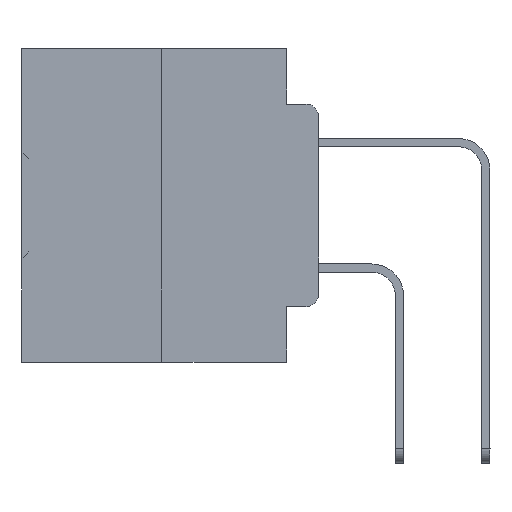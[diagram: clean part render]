
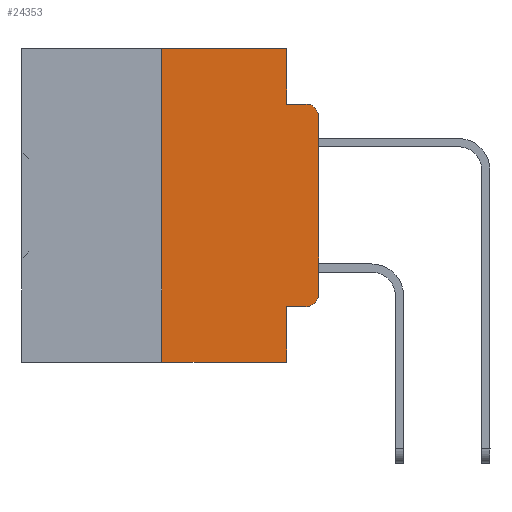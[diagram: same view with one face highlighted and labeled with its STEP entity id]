
A CAD part, left-side view. The second image highlights one B-rep face of the part: STEP entity #24353.
In plain terms, the highlighted planar face has unit normal (-1, 0, 0).
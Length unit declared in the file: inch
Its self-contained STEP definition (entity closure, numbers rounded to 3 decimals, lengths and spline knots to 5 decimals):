
#360 = ORIENTED_EDGE ( 'NONE', *, *, #14744, .F. ) ;
#1172 = ORIENTED_EDGE ( 'NONE', *, *, #17525, .T. ) ;
#1240 = ORIENTED_EDGE ( 'NONE', *, *, #19256, .T. ) ;
#1811 = DIRECTION ( 'NONE',  ( 0., -1., 0. ) ) ;
#2432 = DIRECTION ( 'NONE',  ( 0., 0., -1. ) ) ;
#2628 = ORIENTED_EDGE ( 'NONE', *, *, #6548, .T. ) ;
#3210 = ORIENTED_EDGE ( 'NONE', *, *, #6159, .T. ) ;
#3974 = CARTESIAN_POINT ( 'NONE',  ( 0., 0.051, 0. ) ) ;
#5320 = VERTEX_POINT ( 'NONE', #37767 ) ;
#5536 = VECTOR ( 'NONE', #11918, 39.37008 ) ;
#5666 = AXIS2_PLACEMENT_3D ( 'NONE', #34606, #37260, #12743 ) ;
#6159 = EDGE_CURVE ( 'NONE', #8242, #31587, #16073, .T. ) ;
#6332 = CARTESIAN_POINT ( 'NONE',  ( 0., 0.051, 0. ) ) ;
#6548 = EDGE_CURVE ( 'NONE', #24073, #8242, #27234, .T. ) ;
#6942 = CARTESIAN_POINT ( 'NONE',  ( 0., 0.051, -0.4115 ) ) ;
#7575 = CARTESIAN_POINT ( 'NONE',  ( 0., 0.25, 0. ) ) ;
#8065 = LINE ( 'NONE', #23955, #5536 ) ;
#8242 = VERTEX_POINT ( 'NONE', #32016 ) ;
#8620 = VECTOR ( 'NONE', #15705, 39.37008 ) ;
#9000 = VERTEX_POINT ( 'NONE', #39916 ) ;
#9559 = ORIENTED_EDGE ( 'NONE', *, *, #33309, .F. ) ;
#9646 = VECTOR ( 'NONE', #20033, 39.37008 ) ;
#9676 = CIRCLE ( 'NONE', #37721, 0.02 ) ;
#9790 = DIRECTION ( 'NONE',  ( 0., 0., -1. ) ) ;
#10258 = CARTESIAN_POINT ( 'NONE',  ( 0., 0.051, 0. ) ) ;
#10479 = LINE ( 'NONE', #3974, #38012 ) ;
#11151 = CARTESIAN_POINT ( 'NONE',  ( 0., 0.02, -0.0885 ) ) ;
#11415 = ORIENTED_EDGE ( 'NONE', *, *, #15819, .F. ) ;
#11901 = VERTEX_POINT ( 'NONE', #13279 ) ;
#11918 = DIRECTION ( 'NONE',  ( 0., 0., 1. ) ) ;
#12448 = CARTESIAN_POINT ( 'NONE',  ( 0., 0.02, -0.1085 ) ) ;
#12743 = DIRECTION ( 'NONE',  ( 0., 0., -1. ) ) ;
#13279 = CARTESIAN_POINT ( 'NONE',  ( 0., 0.051, -0.5 ) ) ;
#14744 = EDGE_CURVE ( 'NONE', #30869, #9000, #16304, .T. ) ;
#15273 = CARTESIAN_POINT ( 'NONE',  ( 0., 0., -0.3915 ) ) ;
#15677 = DIRECTION ( 'NONE',  ( 0., -1., 0. ) ) ;
#15705 = DIRECTION ( 'NONE',  ( 0., 0., -1. ) ) ;
#15819 = EDGE_CURVE ( 'NONE', #24073, #11901, #10479, .T. ) ;
#16073 = CIRCLE ( 'NONE', #5666, 0.02 ) ;
#16304 = LINE ( 'NONE', #6332, #8620 ) ;
#17028 = VERTEX_POINT ( 'NONE', #40156 ) ;
#17193 = LINE ( 'NONE', #29066, #34954 ) ;
#17505 = LINE ( 'NONE', #23035, #19625 ) ;
#17525 = EDGE_CURVE ( 'NONE', #31587, #17028, #8065, .T. ) ;
#18326 = VECTOR ( 'NONE', #15677, 39.37008 ) ;
#19256 = EDGE_CURVE ( 'NONE', #27452, #11901, #17193, .T. ) ;
#19332 = VECTOR ( 'NONE', #23729, 39.37008 ) ;
#19625 = VECTOR ( 'NONE', #1811, 39.37008 ) ;
#20033 = DIRECTION ( 'NONE',  ( 0., 0., 1. ) ) ;
#20353 = EDGE_LOOP ( 'NONE', ( #1172, #33511, #40323, #360, #9559, #34715, #1240, #11415, #2628, #3210 ) ) ;
#21201 = DIRECTION ( 'NONE',  ( 1., 0., 0. ) ) ;
#22099 = VERTEX_POINT ( 'NONE', #11151 ) ;
#23035 = CARTESIAN_POINT ( 'NONE',  ( 0., 0.473, 0. ) ) ;
#23729 = DIRECTION ( 'NONE',  ( 0., -1., 0. ) ) ;
#23955 = CARTESIAN_POINT ( 'NONE',  ( 0., 0., 0. ) ) ;
#24073 = VERTEX_POINT ( 'NONE', #6942 ) ;
#24353 = ADVANCED_FACE ( 'NONE', ( #38392 ), #35305, .F. ) ;
#24676 = CARTESIAN_POINT ( 'NONE',  ( 0., 0.051, -0.0885 ) ) ;
#27234 = LINE ( 'NONE', #36403, #19332 ) ;
#27452 = VERTEX_POINT ( 'NONE', #33228 ) ;
#28889 = DIRECTION ( 'NONE',  ( 0., 0., -1. ) ) ;
#29066 = CARTESIAN_POINT ( 'NONE',  ( 0., 0.473, -0.5 ) ) ;
#29199 = CARTESIAN_POINT ( 'NONE',  ( 0., 0.473, 0. ) ) ;
#29661 = DIRECTION ( 'NONE',  ( 0., -1., 0. ) ) ;
#30869 = VERTEX_POINT ( 'NONE', #10258 ) ;
#31556 = EDGE_CURVE ( 'NONE', #9000, #22099, #33677, .T. ) ;
#31587 = VERTEX_POINT ( 'NONE', #15273 ) ;
#32016 = CARTESIAN_POINT ( 'NONE',  ( 0., 0.02, -0.4115 ) ) ;
#33228 = CARTESIAN_POINT ( 'NONE',  ( 0., 0.25, -0.5 ) ) ;
#33309 = EDGE_CURVE ( 'NONE', #5320, #30869, #17505, .T. ) ;
#33511 = ORIENTED_EDGE ( 'NONE', *, *, #37702, .T. ) ;
#33677 = LINE ( 'NONE', #24676, #18326 ) ;
#34606 = CARTESIAN_POINT ( 'NONE',  ( 0., 0.02, -0.3915 ) ) ;
#34715 = ORIENTED_EDGE ( 'NONE', *, *, #37468, .F. ) ;
#34930 = AXIS2_PLACEMENT_3D ( 'NONE', #29199, #21201, #2432 ) ;
#34954 = VECTOR ( 'NONE', #29661, 39.37008 ) ;
#35305 = PLANE ( 'NONE',  #34930 ) ;
#35545 = LINE ( 'NONE', #7575, #9646 ) ;
#36403 = CARTESIAN_POINT ( 'NONE',  ( 0., 0.051, -0.4115 ) ) ;
#37260 = DIRECTION ( 'NONE',  ( -1., 0., 0. ) ) ;
#37468 = EDGE_CURVE ( 'NONE', #27452, #5320, #35545, .T. ) ;
#37570 = DIRECTION ( 'NONE',  ( -1., 0., 0. ) ) ;
#37702 = EDGE_CURVE ( 'NONE', #17028, #22099, #9676, .T. ) ;
#37721 = AXIS2_PLACEMENT_3D ( 'NONE', #12448, #37570, #9790 ) ;
#37767 = CARTESIAN_POINT ( 'NONE',  ( 0., 0.25, 0. ) ) ;
#38012 = VECTOR ( 'NONE', #28889, 39.37008 ) ;
#38392 = FACE_OUTER_BOUND ( 'NONE', #20353, .T. ) ;
#39916 = CARTESIAN_POINT ( 'NONE',  ( 0., 0.051, -0.0885 ) ) ;
#40156 = CARTESIAN_POINT ( 'NONE',  ( 0., 0., -0.1085 ) ) ;
#40323 = ORIENTED_EDGE ( 'NONE', *, *, #31556, .F. ) ;
